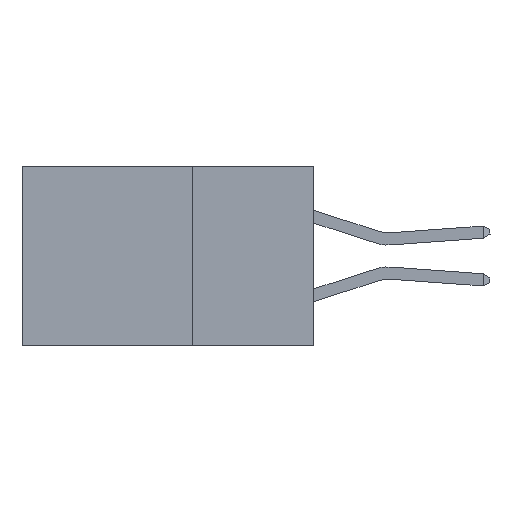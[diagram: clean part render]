
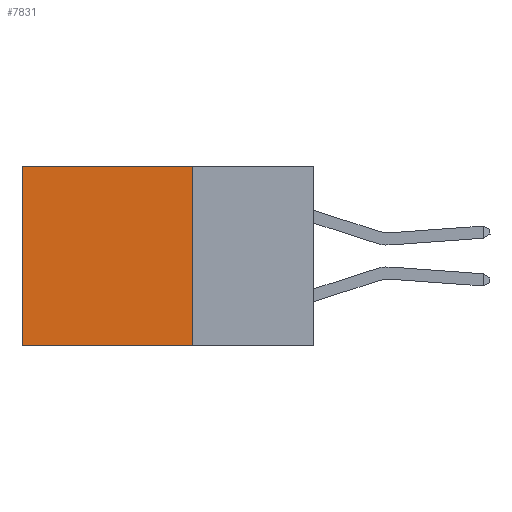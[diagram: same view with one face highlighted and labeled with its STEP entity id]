
A CAD part, left-side view. The second image highlights one B-rep face of the part: STEP entity #7831.
In plain terms, the highlighted planar face has unit normal (-1, 0, 0).
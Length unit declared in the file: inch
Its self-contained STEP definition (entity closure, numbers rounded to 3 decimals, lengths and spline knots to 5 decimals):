
#916 = EDGE_CURVE ( 'NONE', #12128, #5977, #18227, .T. ) ;
#1290 = EDGE_CURVE ( 'NONE', #18144, #5977, #6730, .T. ) ;
#2014 = CARTESIAN_POINT ( 'NONE',  ( 0.2875, 0.25, 0. ) ) ;
#2212 = FACE_OUTER_BOUND ( 'NONE', #13993, .T. ) ;
#3096 = VECTOR ( 'NONE', #3472, 39.37008 ) ;
#3472 = DIRECTION ( 'NONE',  ( 0., 1., 0. ) ) ;
#3667 = CARTESIAN_POINT ( 'NONE',  ( 0.2875, 0.25, 0. ) ) ;
#3843 = VECTOR ( 'NONE', #13837, 39.37008 ) ;
#4142 = VECTOR ( 'NONE', #14055, 39.37008 ) ;
#4679 = CARTESIAN_POINT ( 'NONE',  ( 0.2875, 0.6, -0.37 ) ) ;
#5110 = LINE ( 'NONE', #15623, #4142 ) ;
#5252 = LINE ( 'NONE', #2014, #3096 ) ;
#5407 = PLANE ( 'NONE',  #17980 ) ;
#5796 = ORIENTED_EDGE ( 'NONE', *, *, #6234, .F. ) ;
#5977 = VERTEX_POINT ( 'NONE', #4679 ) ;
#6234 = EDGE_CURVE ( 'NONE', #13475, #12128, #5110, .T. ) ;
#6730 = LINE ( 'NONE', #15414, #3843 ) ;
#7831 = ADVANCED_FACE ( 'NONE', ( #2212 ), #5407, .F. ) ;
#8396 = ORIENTED_EDGE ( 'NONE', *, *, #1290, .T. ) ;
#9532 = CARTESIAN_POINT ( 'NONE',  ( 0.2875, 0.25, 0. ) ) ;
#12128 = VERTEX_POINT ( 'NONE', #16532 ) ;
#13475 = VERTEX_POINT ( 'NONE', #9532 ) ;
#13560 = DIRECTION ( 'NONE',  ( 0., 1., 0. ) ) ;
#13837 = DIRECTION ( 'NONE',  ( 0., 0., -1. ) ) ;
#13993 = EDGE_LOOP ( 'NONE', ( #8396, #18512, #5796, #17468 ) ) ;
#14055 = DIRECTION ( 'NONE',  ( 0., 0., -1. ) ) ;
#14399 = DIRECTION ( 'NONE',  ( 1., 0., 0. ) ) ;
#14645 = VECTOR ( 'NONE', #13560, 39.37008 ) ;
#15414 = CARTESIAN_POINT ( 'NONE',  ( 0.2875, 0.6, 0. ) ) ;
#15623 = CARTESIAN_POINT ( 'NONE',  ( 0.2875, 0.25, 0. ) ) ;
#15771 = EDGE_CURVE ( 'NONE', #13475, #18144, #5252, .T. ) ;
#16532 = CARTESIAN_POINT ( 'NONE',  ( 0.2875, 0.25, -0.37 ) ) ;
#17468 = ORIENTED_EDGE ( 'NONE', *, *, #15771, .T. ) ;
#17505 = DIRECTION ( 'NONE',  ( 0., 0., -1. ) ) ;
#17980 = AXIS2_PLACEMENT_3D ( 'NONE', #3667, #14399, #17505 ) ;
#18135 = CARTESIAN_POINT ( 'NONE',  ( 0.2875, 0.6, 0. ) ) ;
#18144 = VERTEX_POINT ( 'NONE', #18135 ) ;
#18227 = LINE ( 'NONE', #18779, #14645 ) ;
#18512 = ORIENTED_EDGE ( 'NONE', *, *, #916, .F. ) ;
#18779 = CARTESIAN_POINT ( 'NONE',  ( 0.2875, 0.25, -0.37 ) ) ;
